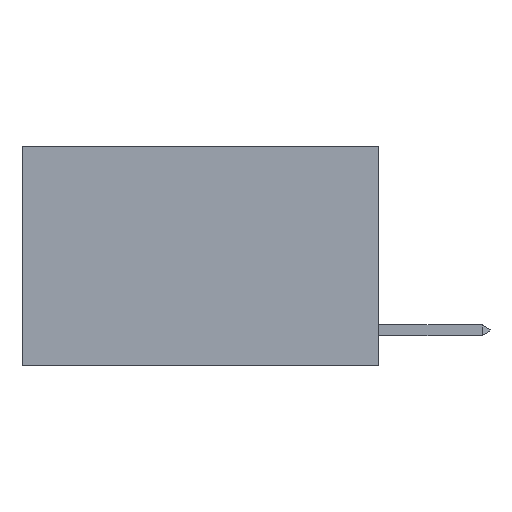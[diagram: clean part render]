
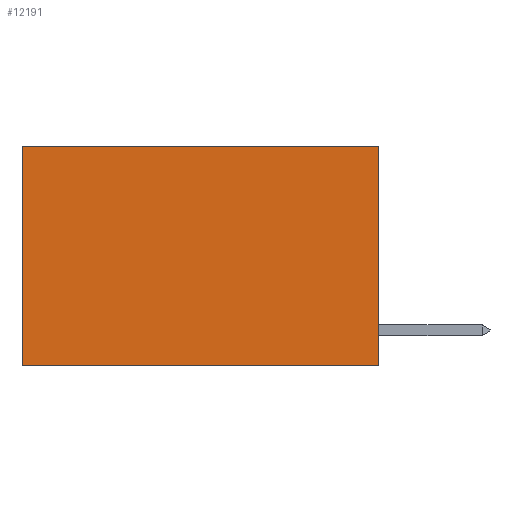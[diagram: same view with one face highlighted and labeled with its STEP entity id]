
A CAD part, left-side view. The second image highlights one B-rep face of the part: STEP entity #12191.
In plain terms, the highlighted planar face has unit normal (-1, 0, 0).
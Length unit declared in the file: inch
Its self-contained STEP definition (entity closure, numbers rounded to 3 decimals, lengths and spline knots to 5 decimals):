
#30 = FACE_OUTER_BOUND ( 'NONE', #16685, .T. ) ;
#377 = EDGE_CURVE ( 'NONE', #18717, #7370, #14437, .T. ) ;
#640 = CARTESIAN_POINT ( 'NONE',  ( 0.2625, 0., -0.37 ) ) ;
#2164 = CARTESIAN_POINT ( 'NONE',  ( 0.2625, 0.6, 0. ) ) ;
#3359 = VECTOR ( 'NONE', #9807, 39.37008 ) ;
#4047 = CARTESIAN_POINT ( 'NONE',  ( 0.2625, 0., 0. ) ) ;
#4290 = EDGE_CURVE ( 'NONE', #7370, #9897, #19299, .T. ) ;
#4412 = EDGE_CURVE ( 'NONE', #9397, #9897, #16922, .T. ) ;
#4625 = CARTESIAN_POINT ( 'NONE',  ( 0.2625, 0., -0.37 ) ) ;
#4811 = ORIENTED_EDGE ( 'NONE', *, *, #4412, .F. ) ;
#5165 = VECTOR ( 'NONE', #9510, 39.37008 ) ;
#5887 = ORIENTED_EDGE ( 'NONE', *, *, #4290, .T. ) ;
#6433 = VECTOR ( 'NONE', #15984, 39.37008 ) ;
#7020 = LINE ( 'NONE', #4047, #11598 ) ;
#7370 = VERTEX_POINT ( 'NONE', #2164 ) ;
#7778 = CARTESIAN_POINT ( 'NONE',  ( 0.2625, 0.6, 0. ) ) ;
#8015 = ORIENTED_EDGE ( 'NONE', *, *, #377, .T. ) ;
#8318 = DIRECTION ( 'NONE',  ( 1., 0., 0. ) ) ;
#8825 = CARTESIAN_POINT ( 'NONE',  ( 0.2625, 0.6, -0.37 ) ) ;
#9397 = VERTEX_POINT ( 'NONE', #640 ) ;
#9510 = DIRECTION ( 'NONE',  ( 0., 0., -1. ) ) ;
#9807 = DIRECTION ( 'NONE',  ( 0., 1., 0. ) ) ;
#9897 = VERTEX_POINT ( 'NONE', #8825 ) ;
#10399 = AXIS2_PLACEMENT_3D ( 'NONE', #11699, #8318, #20198 ) ;
#11598 = VECTOR ( 'NONE', #14251, 39.37008 ) ;
#11699 = CARTESIAN_POINT ( 'NONE',  ( 0.2625, 0., 0. ) ) ;
#12191 = ADVANCED_FACE ( 'NONE', ( #30 ), #18426, .F. ) ;
#12842 = ORIENTED_EDGE ( 'NONE', *, *, #16569, .F. ) ;
#14251 = DIRECTION ( 'NONE',  ( 0., 0., -1. ) ) ;
#14437 = LINE ( 'NONE', #17738, #6433 ) ;
#15984 = DIRECTION ( 'NONE',  ( 0., 1., 0. ) ) ;
#16569 = EDGE_CURVE ( 'NONE', #18717, #9397, #7020, .T. ) ;
#16685 = EDGE_LOOP ( 'NONE', ( #5887, #4811, #12842, #8015 ) ) ;
#16922 = LINE ( 'NONE', #4625, #3359 ) ;
#17738 = CARTESIAN_POINT ( 'NONE',  ( 0.2625, 0., 0. ) ) ;
#18191 = CARTESIAN_POINT ( 'NONE',  ( 0.2625, 0., 0. ) ) ;
#18426 = PLANE ( 'NONE',  #10399 ) ;
#18717 = VERTEX_POINT ( 'NONE', #18191 ) ;
#19299 = LINE ( 'NONE', #7778, #5165 ) ;
#20198 = DIRECTION ( 'NONE',  ( 0., 0., -1. ) ) ;
